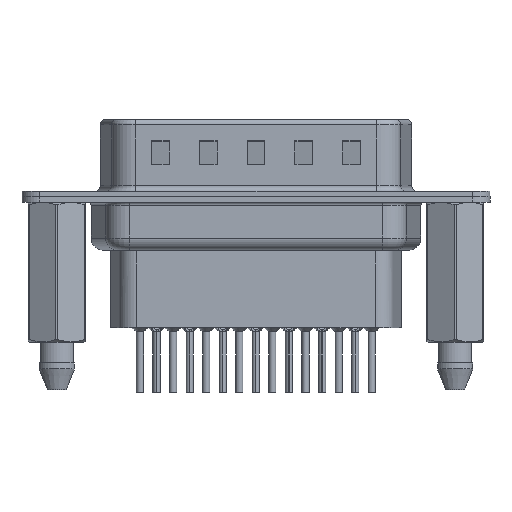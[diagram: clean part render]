
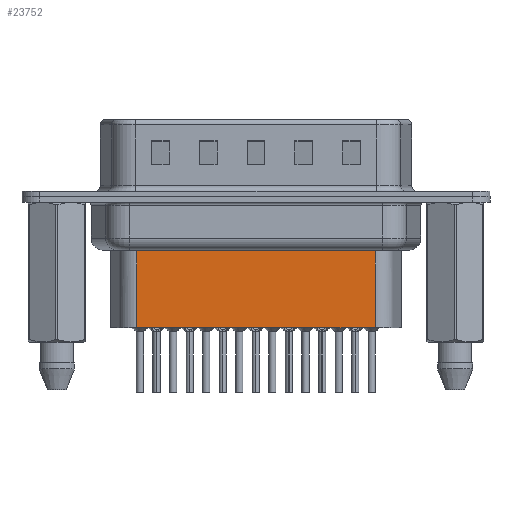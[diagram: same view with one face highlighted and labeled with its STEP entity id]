
A CAD part, front view. The second image highlights one B-rep face of the part: STEP entity #23752.
In plain terms, the highlighted planar face has unit normal (0, -1, 0).
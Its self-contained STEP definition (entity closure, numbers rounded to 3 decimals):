
#647 = VERTEX_POINT ( 'NONE', #3818 ) ;
#1106 = CARTESIAN_POINT ( 'NONE',  ( 6.434, -3.5, -4.097 ) ) ;
#2552 = VERTEX_POINT ( 'NONE', #12145 ) ;
#2634 = EDGE_CURVE ( 'NONE', #23232, #647, #13957, .T. ) ;
#2832 = VECTOR ( 'NONE', #15673, 1000. ) ;
#2948 = DIRECTION ( 'NONE',  ( -1., 0., 0. ) ) ;
#3800 = EDGE_CURVE ( 'NONE', #2552, #18074, #6440, .T. ) ;
#3818 = CARTESIAN_POINT ( 'NONE',  ( 6.681, -3.5, -4.097 ) ) ;
#4027 = ORIENTED_EDGE ( 'NONE', *, *, #2634, .T. ) ;
#4091 = EDGE_CURVE ( 'NONE', #647, #18074, #22868, .T. ) ;
#5195 = DIRECTION ( 'NONE',  ( 1., 0., 0. ) ) ;
#5292 = DIRECTION ( 'NONE',  ( 0., 0., -1. ) ) ;
#5542 = DIRECTION ( 'NONE',  ( 0., -1., 0. ) ) ;
#6440 = LINE ( 'NONE', #19840, #8608 ) ;
#7619 = ORIENTED_EDGE ( 'NONE', *, *, #20783, .F. ) ;
#8608 = VECTOR ( 'NONE', #2948, 1000. ) ;
#9410 = CARTESIAN_POINT ( 'NONE',  ( 26.619, -3.5, -3.1 ) ) ;
#10779 = PLANE ( 'NONE',  #19148 ) ;
#12145 = CARTESIAN_POINT ( 'NONE',  ( 26.619, -3.5, -10.95 ) ) ;
#13957 = LINE ( 'NONE', #1106, #2832 ) ;
#14459 = CARTESIAN_POINT ( 'NONE',  ( 26.619, -3.5, -4.097 ) ) ;
#14925 = CARTESIAN_POINT ( 'NONE',  ( 6.681, -3.5, -3.1 ) ) ;
#15673 = DIRECTION ( 'NONE',  ( -1., 0., 0. ) ) ;
#17615 = ORIENTED_EDGE ( 'NONE', *, *, #4091, .T. ) ;
#18074 = VERTEX_POINT ( 'NONE', #21837 ) ;
#19148 = AXIS2_PLACEMENT_3D ( 'NONE', #23946, #5542, #5195 ) ;
#19486 = VECTOR ( 'NONE', #22389, 1000. ) ;
#19840 = CARTESIAN_POINT ( 'NONE',  ( 6.681, -3.5, -10.95 ) ) ;
#20783 = EDGE_CURVE ( 'NONE', #23232, #2552, #23924, .T. ) ;
#21115 = VECTOR ( 'NONE', #5292, 1000. ) ;
#21837 = CARTESIAN_POINT ( 'NONE',  ( 6.681, -3.5, -10.95 ) ) ;
#22023 = EDGE_LOOP ( 'NONE', ( #7619, #4027, #17615, #22467 ) ) ;
#22389 = DIRECTION ( 'NONE',  ( 0., 0., -1. ) ) ;
#22467 = ORIENTED_EDGE ( 'NONE', *, *, #3800, .F. ) ;
#22868 = LINE ( 'NONE', #14925, #19486 ) ;
#23232 = VERTEX_POINT ( 'NONE', #14459 ) ;
#23707 = FACE_OUTER_BOUND ( 'NONE', #22023, .T. ) ;
#23752 = ADVANCED_FACE ( 'NONE', ( #23707 ), #10779, .T. ) ;
#23924 = LINE ( 'NONE', #9410, #21115 ) ;
#23946 = CARTESIAN_POINT ( 'NONE',  ( 6.681, -3.5, -3.1 ) ) ;
